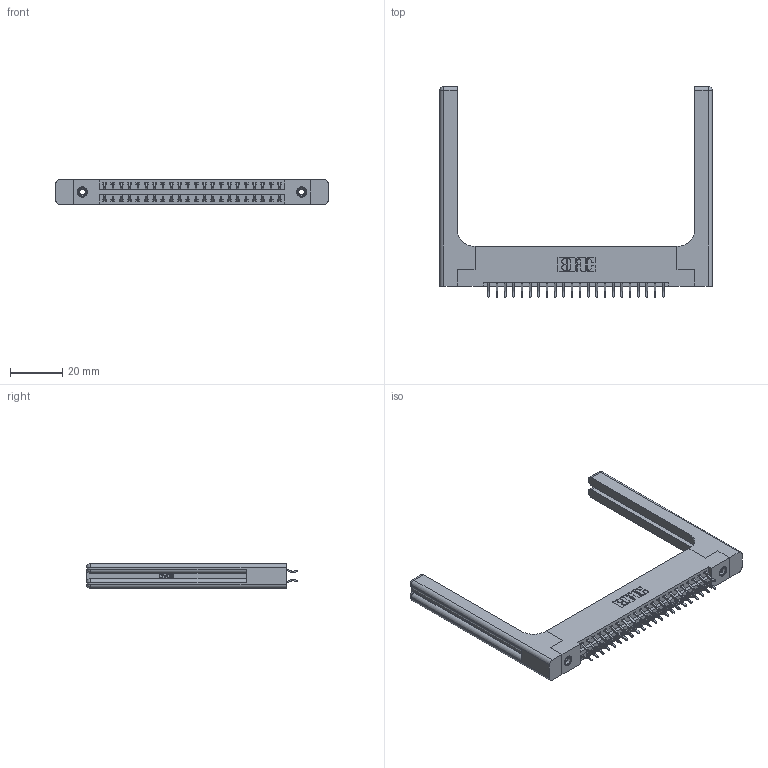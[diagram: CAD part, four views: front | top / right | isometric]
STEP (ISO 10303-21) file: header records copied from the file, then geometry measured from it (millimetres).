
FILE_DESCRIPTION (( 'STEP AP203' ), '1' );
FILE_NAME ('396-044-556-258.STEP', '2019-10-30T11:41:28', ( '' ), ( '' ), 'SwSTEP 2.0', 'SolidWorks 2016', '' );
FILE_SCHEMA (( 'CONFIG_CONTROL_DESIGN' ));
Length unit declared in the file: inch
Products named in the file (5): 345-292-001_556 Tail; 396-044-556-258; 345-250-001_345-250-001-102; 346-220-058_345-220-058; 346 Part_Flush Mounting Lugs - 0.156 Dia-TH
Assembly tree (49 placements, depth 2):
  396-044-556-258
    346 Part_Flush Mounting Lugs - 0.156 Dia-TH
    345-292-001_556 Tail  x44
    345-250-001_345-250-001-102  x2
    346-220-058_345-220-058  x2
Bounding box: 103.91 x 80.53 x 9.4 mm (x, y, z)
Volume: 17469.8 mm3; surface area: 18329.6 mm2
Topology: 49 solids, 49 shells, 2930 faces, 8607 edges, 5658 vertices
Faces by surface type: plane 1940, cylinder 930, bspline 36, cone 12, sphere 8, torus 4
Entity records: 22452 total; most frequent: CARTESIAN_POINT 4749, ORIENTED_EDGE 3468, DIRECTION 3158, EDGE_CURVE 1734, VECTOR 1414, LINE 1414, VERTEX_POINT 1146, AXIS2_PLACEMENT_3D 872
